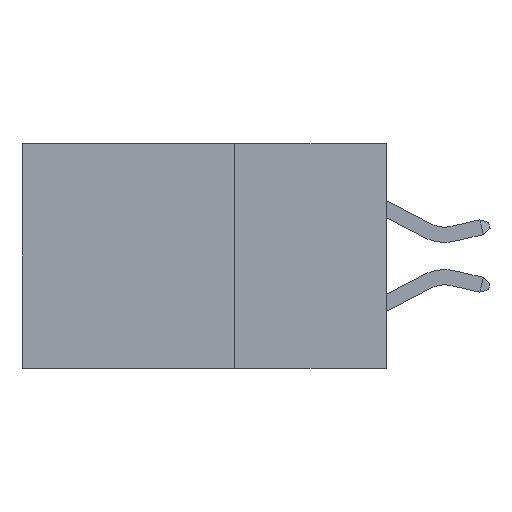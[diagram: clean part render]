
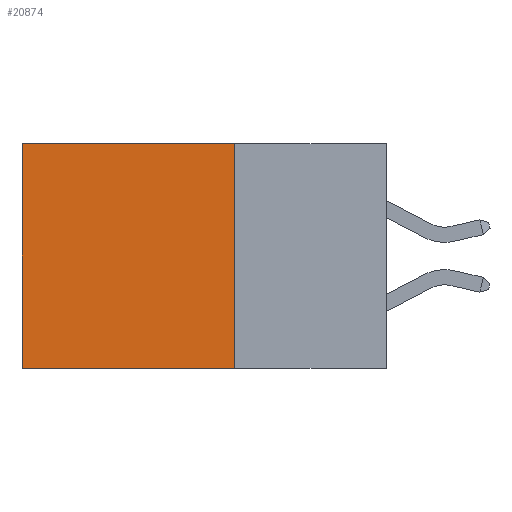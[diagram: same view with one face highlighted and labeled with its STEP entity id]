
A CAD part, left-side view. The second image highlights one B-rep face of the part: STEP entity #20874.
In plain terms, the highlighted planar face has unit normal (-1, 0, 0).
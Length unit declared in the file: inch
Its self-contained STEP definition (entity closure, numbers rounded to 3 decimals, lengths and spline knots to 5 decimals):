
#1063 = LINE ( 'NONE', #14246, #18603 ) ;
#2212 = VECTOR ( 'NONE', #27113, 39.37008 ) ;
#2217 = EDGE_CURVE ( 'NONE', #22838, #9521, #1063, .T. ) ;
#2695 = DIRECTION ( 'NONE',  ( 1., 0., 0. ) ) ;
#2978 = LINE ( 'NONE', #18060, #2212 ) ;
#4518 = LINE ( 'NONE', #10321, #11317 ) ;
#4848 = EDGE_CURVE ( 'NONE', #19543, #28241, #4518, .T. ) ;
#4911 = CARTESIAN_POINT ( 'NONE',  ( 0.298, 0.25, 0. ) ) ;
#5012 = DIRECTION ( 'NONE',  ( 0., 0., -1. ) ) ;
#5039 = EDGE_CURVE ( 'NONE', #19543, #22838, #14527, .T. ) ;
#6504 = EDGE_CURVE ( 'NONE', #28241, #9521, #2978, .T. ) ;
#8610 = ORIENTED_EDGE ( 'NONE', *, *, #2217, .T. ) ;
#9521 = VERTEX_POINT ( 'NONE', #17697 ) ;
#9563 = CARTESIAN_POINT ( 'NONE',  ( 0.298, 0.25, 0. ) ) ;
#10321 = CARTESIAN_POINT ( 'NONE',  ( 0.298, 0.25, 0. ) ) ;
#11053 = ORIENTED_EDGE ( 'NONE', *, *, #5039, .T. ) ;
#11317 = VECTOR ( 'NONE', #21589, 39.37008 ) ;
#13485 = CARTESIAN_POINT ( 'NONE',  ( 0.298, 0.25, 0. ) ) ;
#13809 = VECTOR ( 'NONE', #18256, 39.37008 ) ;
#14246 = CARTESIAN_POINT ( 'NONE',  ( 0.298, 0.6, 0. ) ) ;
#14527 = LINE ( 'NONE', #13485, #13809 ) ;
#15897 = ORIENTED_EDGE ( 'NONE', *, *, #6504, .F. ) ;
#17697 = CARTESIAN_POINT ( 'NONE',  ( 0.298, 0.6, -0.37 ) ) ;
#18060 = CARTESIAN_POINT ( 'NONE',  ( 0.298, 0.25, -0.37 ) ) ;
#18256 = DIRECTION ( 'NONE',  ( 0., 1., 0. ) ) ;
#18603 = VECTOR ( 'NONE', #18841, 39.37008 ) ;
#18749 = CARTESIAN_POINT ( 'NONE',  ( 0.298, 0.25, -0.37 ) ) ;
#18841 = DIRECTION ( 'NONE',  ( 0., 0., -1. ) ) ;
#19543 = VERTEX_POINT ( 'NONE', #9563 ) ;
#20874 = ADVANCED_FACE ( 'NONE', ( #25270 ), #21959, .F. ) ;
#21589 = DIRECTION ( 'NONE',  ( 0., 0., -1. ) ) ;
#21959 = PLANE ( 'NONE',  #24989 ) ;
#22838 = VERTEX_POINT ( 'NONE', #26771 ) ;
#24989 = AXIS2_PLACEMENT_3D ( 'NONE', #4911, #2695, #5012 ) ;
#25270 = FACE_OUTER_BOUND ( 'NONE', #27933, .T. ) ;
#25393 = ORIENTED_EDGE ( 'NONE', *, *, #4848, .F. ) ;
#26771 = CARTESIAN_POINT ( 'NONE',  ( 0.298, 0.6, 0. ) ) ;
#27113 = DIRECTION ( 'NONE',  ( 0., 1., 0. ) ) ;
#27933 = EDGE_LOOP ( 'NONE', ( #8610, #15897, #25393, #11053 ) ) ;
#28241 = VERTEX_POINT ( 'NONE', #18749 ) ;
